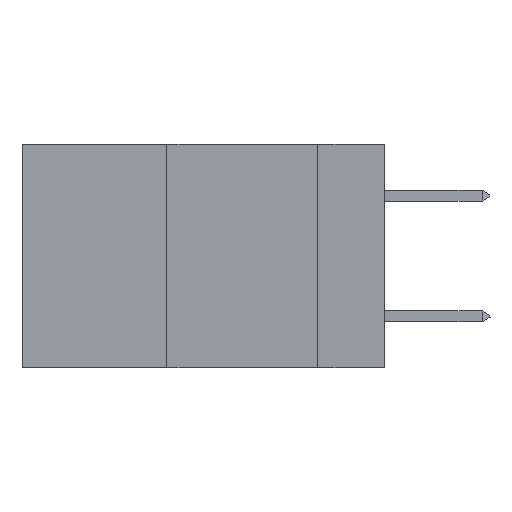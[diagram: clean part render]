
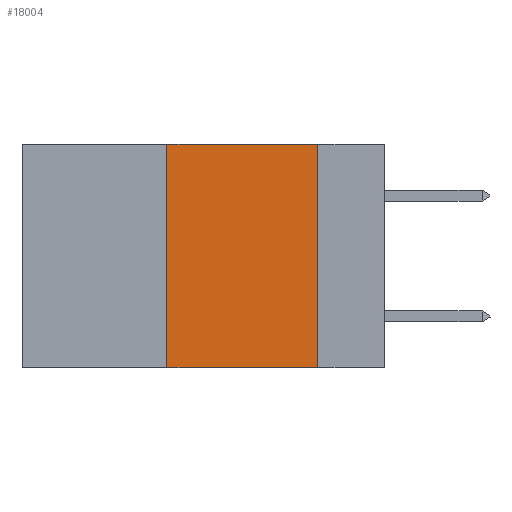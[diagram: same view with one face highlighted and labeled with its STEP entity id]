
A CAD part, left-side view. The second image highlights one B-rep face of the part: STEP entity #18004.
In plain terms, the highlighted planar face has unit normal (-1, 0, 0).
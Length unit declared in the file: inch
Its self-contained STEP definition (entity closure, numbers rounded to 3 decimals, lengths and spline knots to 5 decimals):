
#679 = PLANE ( 'NONE',  #15405 ) ;
#1620 = LINE ( 'NONE', #17220, #14219 ) ;
#2013 = EDGE_CURVE ( 'NONE', #7456, #15961, #20103, .T. ) ;
#2181 = ORIENTED_EDGE ( 'NONE', *, *, #3674, .F. ) ;
#3270 = DIRECTION ( 'NONE',  ( 0., 0., 1. ) ) ;
#3309 = CARTESIAN_POINT ( 'NONE',  ( 0., 0.11, -0.37 ) ) ;
#3674 = EDGE_CURVE ( 'NONE', #15961, #19141, #4225, .T. ) ;
#3882 = CARTESIAN_POINT ( 'NONE',  ( 0., 0.6, 0. ) ) ;
#4225 = LINE ( 'NONE', #3882, #8481 ) ;
#4285 = CARTESIAN_POINT ( 'NONE',  ( 0., 0.36, 0. ) ) ;
#4450 = VERTEX_POINT ( 'NONE', #3309 ) ;
#4908 = EDGE_CURVE ( 'NONE', #19141, #4450, #1620, .T. ) ;
#6975 = CARTESIAN_POINT ( 'NONE',  ( 0., 0.11, 0. ) ) ;
#7105 = CARTESIAN_POINT ( 'NONE',  ( 0., 0.6, 0. ) ) ;
#7339 = DIRECTION ( 'NONE',  ( 0., -1., 0. ) ) ;
#7456 = VERTEX_POINT ( 'NONE', #9496 ) ;
#8481 = VECTOR ( 'NONE', #19978, 39.37008 ) ;
#8695 = DIRECTION ( 'NONE',  ( 1., 0., 0. ) ) ;
#9496 = CARTESIAN_POINT ( 'NONE',  ( 0., 0.36, -0.37 ) ) ;
#10436 = EDGE_CURVE ( 'NONE', #7456, #4450, #12994, .T. ) ;
#10730 = ORIENTED_EDGE ( 'NONE', *, *, #10436, .T. ) ;
#11238 = FACE_OUTER_BOUND ( 'NONE', #19830, .T. ) ;
#12340 = CARTESIAN_POINT ( 'NONE',  ( 0., 0.36, 0. ) ) ;
#12994 = LINE ( 'NONE', #13647, #16509 ) ;
#13647 = CARTESIAN_POINT ( 'NONE',  ( 0., 0.6, -0.37 ) ) ;
#14205 = DIRECTION ( 'NONE',  ( 0., 0., -1. ) ) ;
#14219 = VECTOR ( 'NONE', #14205, 39.37008 ) ;
#15266 = ORIENTED_EDGE ( 'NONE', *, *, #2013, .F. ) ;
#15405 = AXIS2_PLACEMENT_3D ( 'NONE', #7105, #8695, #18400 ) ;
#15961 = VERTEX_POINT ( 'NONE', #12340 ) ;
#16509 = VECTOR ( 'NONE', #7339, 39.37008 ) ;
#17220 = CARTESIAN_POINT ( 'NONE',  ( 0., 0.11, 0. ) ) ;
#17322 = VECTOR ( 'NONE', #3270, 39.37008 ) ;
#18004 = ADVANCED_FACE ( 'NONE', ( #11238 ), #679, .F. ) ;
#18400 = DIRECTION ( 'NONE',  ( 0., 0., -1. ) ) ;
#18823 = ORIENTED_EDGE ( 'NONE', *, *, #4908, .F. ) ;
#19141 = VERTEX_POINT ( 'NONE', #6975 ) ;
#19830 = EDGE_LOOP ( 'NONE', ( #18823, #2181, #15266, #10730 ) ) ;
#19978 = DIRECTION ( 'NONE',  ( 0., -1., 0. ) ) ;
#20103 = LINE ( 'NONE', #4285, #17322 ) ;
